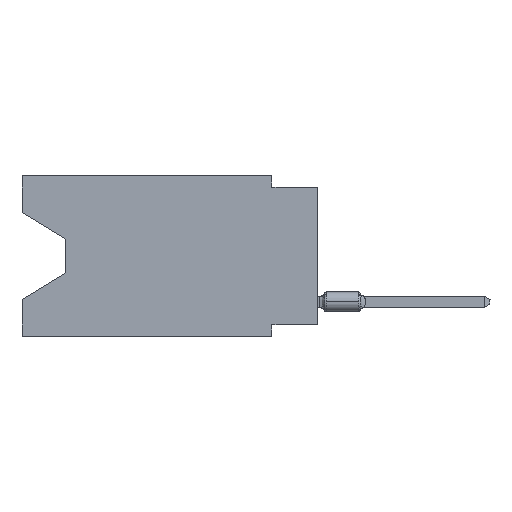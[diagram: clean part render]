
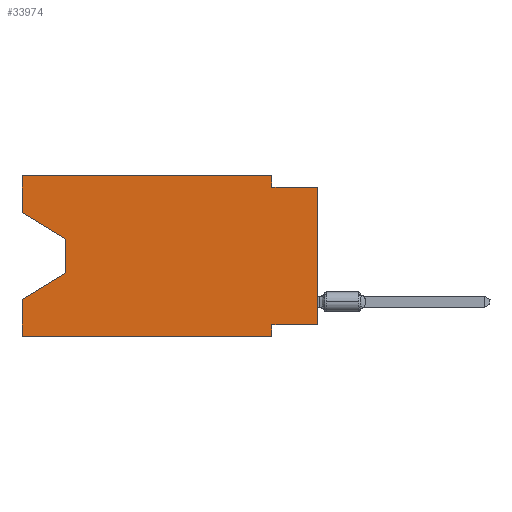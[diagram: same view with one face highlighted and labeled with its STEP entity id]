
A CAD part, left-side view. The second image highlights one B-rep face of the part: STEP entity #33974.
In plain terms, the highlighted planar face has unit normal (-1, 0, 0).
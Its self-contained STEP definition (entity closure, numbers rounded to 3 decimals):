
#230 = ORIENTED_EDGE ( 'NONE', *, *, #7068, .F. ) ;
#242 = CARTESIAN_POINT ( 'NONE',  ( 0., 16.383, -6.852 ) ) ;
#1060 = ORIENTED_EDGE ( 'NONE', *, *, #9881, .F. ) ;
#2253 = CARTESIAN_POINT ( 'NONE',  ( 0., 2.54, 0. ) ) ;
#2786 = EDGE_LOOP ( 'NONE', ( #32330, #69833, #4574, #93438, #58833, #230, #31467, #26826, #14972, #1060, #76952, #30181 ) ) ;
#4356 = EDGE_CURVE ( 'NONE', #44840, #12991, #9844, .T. ) ;
#4574 = ORIENTED_EDGE ( 'NONE', *, *, #74840, .T. ) ;
#4653 = CARTESIAN_POINT ( 'NONE',  ( 0., 16.383, 0. ) ) ;
#5356 = DIRECTION ( 'NONE',  ( 0., 0., -1. ) ) ;
#7068 = EDGE_CURVE ( 'NONE', #108951, #10734, #28386, .T. ) ;
#7282 = CARTESIAN_POINT ( 'NONE',  ( 0., 13.97, -3.505 ) ) ;
#8012 = DIRECTION ( 'NONE',  ( 0., -1., 0. ) ) ;
#8590 = VERTEX_POINT ( 'NONE', #104522 ) ;
#9844 = LINE ( 'NONE', #45258, #39750 ) ;
#9881 = EDGE_CURVE ( 'NONE', #17041, #70619, #97541, .T. ) ;
#10734 = VERTEX_POINT ( 'NONE', #70436 ) ;
#10739 = VECTOR ( 'NONE', #69696, 1000. ) ;
#10850 = VECTOR ( 'NONE', #45781, 1000. ) ;
#11585 = LINE ( 'NONE', #54580, #63782 ) ;
#12991 = VERTEX_POINT ( 'NONE', #55956 ) ;
#14972 = ORIENTED_EDGE ( 'NONE', *, *, #81929, .F. ) ;
#16735 = LINE ( 'NONE', #104395, #41350 ) ;
#17041 = VERTEX_POINT ( 'NONE', #2253 ) ;
#17285 = CARTESIAN_POINT ( 'NONE',  ( 0., 16.383, 0. ) ) ;
#20272 = LINE ( 'NONE', #46413, #76264 ) ;
#21949 = EDGE_CURVE ( 'NONE', #103246, #108951, #20272, .T. ) ;
#26826 = ORIENTED_EDGE ( 'NONE', *, *, #61535, .T. ) ;
#27530 = EDGE_CURVE ( 'NONE', #44659, #90569, #104898, .T. ) ;
#27881 = DIRECTION ( 'NONE',  ( 0., -0.855, -0.519 ) ) ;
#28386 = LINE ( 'NONE', #90488, #94011 ) ;
#30181 = ORIENTED_EDGE ( 'NONE', *, *, #51043, .F. ) ;
#30529 = CARTESIAN_POINT ( 'NONE',  ( 0., 16.383, -8.89 ) ) ;
#31467 = ORIENTED_EDGE ( 'NONE', *, *, #21949, .F. ) ;
#31629 = VERTEX_POINT ( 'NONE', #38331 ) ;
#31989 = VERTEX_POINT ( 'NONE', #81190 ) ;
#32330 = ORIENTED_EDGE ( 'NONE', *, *, #75745, .T. ) ;
#32369 = DIRECTION ( 'NONE',  ( 0., -1., 0. ) ) ;
#33974 = ADVANCED_FACE ( 'NONE', ( #111007 ), #102294, .F. ) ;
#38331 = CARTESIAN_POINT ( 'NONE',  ( 0., 16.383, -2.038 ) ) ;
#38370 = VECTOR ( 'NONE', #8012, 1000. ) ;
#39750 = VECTOR ( 'NONE', #80652, 1000. ) ;
#41350 = VECTOR ( 'NONE', #60269, 1000. ) ;
#44659 = VERTEX_POINT ( 'NONE', #30529 ) ;
#44780 = AXIS2_PLACEMENT_3D ( 'NONE', #85454, #103439, #5356 ) ;
#44840 = VERTEX_POINT ( 'NONE', #7282 ) ;
#45258 = CARTESIAN_POINT ( 'NONE',  ( 0., 13.97, -3.505 ) ) ;
#45781 = DIRECTION ( 'NONE',  ( 0., 0., 1. ) ) ;
#46413 = CARTESIAN_POINT ( 'NONE',  ( 0., 0., -8.255 ) ) ;
#47307 = CARTESIAN_POINT ( 'NONE',  ( 0., 2.54, -0.635 ) ) ;
#51043 = EDGE_CURVE ( 'NONE', #31629, #8590, #74180, .T. ) ;
#51142 = EDGE_CURVE ( 'NONE', #44659, #10734, #111328, .T. ) ;
#54580 = CARTESIAN_POINT ( 'NONE',  ( 0., 16.383, -2.038 ) ) ;
#55696 = DIRECTION ( 'NONE',  ( 0., 1., 0. ) ) ;
#55956 = CARTESIAN_POINT ( 'NONE',  ( 0., 13.97, -5.385 ) ) ;
#57106 = LINE ( 'NONE', #91923, #75353 ) ;
#58833 = ORIENTED_EDGE ( 'NONE', *, *, #51142, .T. ) ;
#60201 = VECTOR ( 'NONE', #77991, 1000. ) ;
#60269 = DIRECTION ( 'NONE',  ( 0., 0.855, -0.519 ) ) ;
#61535 = EDGE_CURVE ( 'NONE', #103246, #31989, #103544, .T. ) ;
#63782 = VECTOR ( 'NONE', #27881, 1000. ) ;
#64652 = DIRECTION ( 'NONE',  ( 0., -1., 0. ) ) ;
#65656 = EDGE_CURVE ( 'NONE', #8590, #17041, #96816, .T. ) ;
#69696 = DIRECTION ( 'NONE',  ( 0., 0., -1. ) ) ;
#69833 = ORIENTED_EDGE ( 'NONE', *, *, #4356, .T. ) ;
#70436 = CARTESIAN_POINT ( 'NONE',  ( 0., 2.54, -8.89 ) ) ;
#70619 = VERTEX_POINT ( 'NONE', #47307 ) ;
#74180 = LINE ( 'NONE', #89902, #10850 ) ;
#74840 = EDGE_CURVE ( 'NONE', #12991, #90569, #16735, .T. ) ;
#75353 = VECTOR ( 'NONE', #64652, 1000. ) ;
#75745 = EDGE_CURVE ( 'NONE', #31629, #44840, #11585, .T. ) ;
#76264 = VECTOR ( 'NONE', #55696, 1000. ) ;
#76952 = ORIENTED_EDGE ( 'NONE', *, *, #65656, .F. ) ;
#77047 = CARTESIAN_POINT ( 'NONE',  ( 0., 16.383, -8.89 ) ) ;
#77991 = DIRECTION ( 'NONE',  ( 0., 0., 1. ) ) ;
#80652 = DIRECTION ( 'NONE',  ( 0., 0., -1. ) ) ;
#81190 = CARTESIAN_POINT ( 'NONE',  ( 0., 0., -0.635 ) ) ;
#81781 = DIRECTION ( 'NONE',  ( 0., 0., -1. ) ) ;
#81929 = EDGE_CURVE ( 'NONE', #70619, #31989, #57106, .T. ) ;
#85454 = CARTESIAN_POINT ( 'NONE',  ( 0., 16.383, 0. ) ) ;
#86691 = VECTOR ( 'NONE', #92301, 1000. ) ;
#86887 = CARTESIAN_POINT ( 'NONE',  ( 0., 2.54, -8.255 ) ) ;
#87834 = CARTESIAN_POINT ( 'NONE',  ( 0., 0., 0. ) ) ;
#89902 = CARTESIAN_POINT ( 'NONE',  ( 0., 16.383, 0. ) ) ;
#90488 = CARTESIAN_POINT ( 'NONE',  ( 0., 2.54, -8.89 ) ) ;
#90569 = VERTEX_POINT ( 'NONE', #242 ) ;
#91923 = CARTESIAN_POINT ( 'NONE',  ( 0., 0., -0.635 ) ) ;
#92301 = DIRECTION ( 'NONE',  ( 0., 0., 1. ) ) ;
#93438 = ORIENTED_EDGE ( 'NONE', *, *, #27530, .F. ) ;
#94011 = VECTOR ( 'NONE', #81781, 1000. ) ;
#96816 = LINE ( 'NONE', #17285, #38370 ) ;
#97498 = CARTESIAN_POINT ( 'NONE',  ( 0., 0., -8.255 ) ) ;
#97541 = LINE ( 'NONE', #105685, #10739 ) ;
#101648 = VECTOR ( 'NONE', #32369, 1000. ) ;
#102294 = PLANE ( 'NONE',  #44780 ) ;
#103246 = VERTEX_POINT ( 'NONE', #97498 ) ;
#103439 = DIRECTION ( 'NONE',  ( 1., 0., 0. ) ) ;
#103544 = LINE ( 'NONE', #87834, #60201 ) ;
#104395 = CARTESIAN_POINT ( 'NONE',  ( 0., 13.97, -5.385 ) ) ;
#104522 = CARTESIAN_POINT ( 'NONE',  ( 0., 16.383, 0. ) ) ;
#104898 = LINE ( 'NONE', #4653, #86691 ) ;
#105685 = CARTESIAN_POINT ( 'NONE',  ( 0., 2.54, 0. ) ) ;
#108951 = VERTEX_POINT ( 'NONE', #86887 ) ;
#111007 = FACE_OUTER_BOUND ( 'NONE', #2786, .T. ) ;
#111328 = LINE ( 'NONE', #77047, #101648 ) ;
